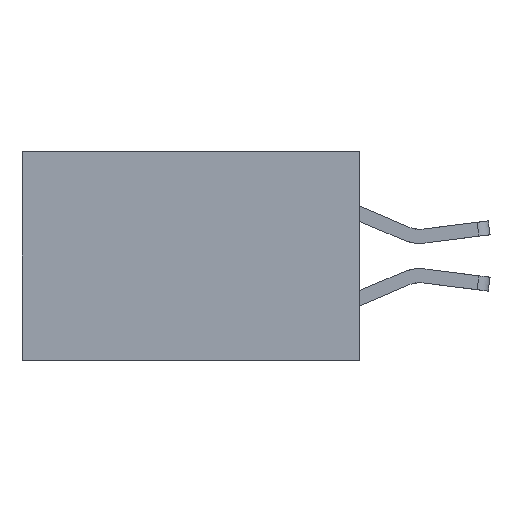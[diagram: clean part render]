
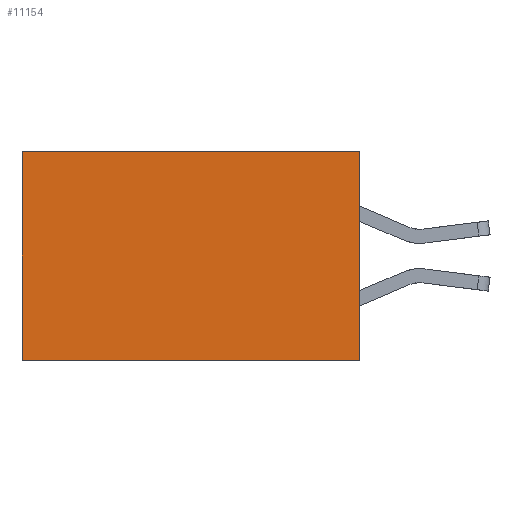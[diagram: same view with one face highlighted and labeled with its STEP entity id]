
A CAD part, left-side view. The second image highlights one B-rep face of the part: STEP entity #11154.
In plain terms, the highlighted planar face has unit normal (-1, 0, 0).
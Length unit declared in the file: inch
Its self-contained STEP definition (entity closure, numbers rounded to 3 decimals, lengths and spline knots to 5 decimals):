
#150 = DIRECTION ( 'NONE',  ( 0., 0., -1. ) ) ;
#681 = EDGE_LOOP ( 'NONE', ( #3591, #5218, #7576, #5569 ) ) ;
#901 = CARTESIAN_POINT ( 'NONE',  ( 0.2875, 0., 0. ) ) ;
#1009 = CARTESIAN_POINT ( 'NONE',  ( 0.2875, 0., 0. ) ) ;
#1150 = VECTOR ( 'NONE', #8488, 39.37008 ) ;
#2266 = DIRECTION ( 'NONE',  ( 0., 0., -1. ) ) ;
#2392 = VECTOR ( 'NONE', #3498, 39.37008 ) ;
#3498 = DIRECTION ( 'NONE',  ( 0., 1., 0. ) ) ;
#3591 = ORIENTED_EDGE ( 'NONE', *, *, #5013, .T. ) ;
#4480 = CARTESIAN_POINT ( 'NONE',  ( 0.2875, 0., -0.37 ) ) ;
#4952 = VERTEX_POINT ( 'NONE', #4480 ) ;
#5013 = EDGE_CURVE ( 'NONE', #6697, #14287, #14569, .T. ) ;
#5218 = ORIENTED_EDGE ( 'NONE', *, *, #15035, .F. ) ;
#5569 = ORIENTED_EDGE ( 'NONE', *, *, #9797, .T. ) ;
#5735 = LINE ( 'NONE', #8496, #11167 ) ;
#6097 = LINE ( 'NONE', #9530, #2392 ) ;
#6520 = CARTESIAN_POINT ( 'NONE',  ( 0.2875, 0., 0. ) ) ;
#6697 = VERTEX_POINT ( 'NONE', #12392 ) ;
#6992 = EDGE_CURVE ( 'NONE', #13157, #4952, #11507, .T. ) ;
#7576 = ORIENTED_EDGE ( 'NONE', *, *, #6992, .F. ) ;
#7700 = DIRECTION ( 'NONE',  ( 1., 0., 0. ) ) ;
#8488 = DIRECTION ( 'NONE',  ( 0., 0., -1. ) ) ;
#8496 = CARTESIAN_POINT ( 'NONE',  ( 0.2875, 0., -0.37 ) ) ;
#9530 = CARTESIAN_POINT ( 'NONE',  ( 0.2875, 0., 0. ) ) ;
#9797 = EDGE_CURVE ( 'NONE', #13157, #6697, #6097, .T. ) ;
#10917 = AXIS2_PLACEMENT_3D ( 'NONE', #6520, #7700, #150 ) ;
#11154 = ADVANCED_FACE ( 'NONE', ( #13433 ), #13381, .F. ) ;
#11167 = VECTOR ( 'NONE', #14165, 39.37008 ) ;
#11507 = LINE ( 'NONE', #901, #14167 ) ;
#11859 = CARTESIAN_POINT ( 'NONE',  ( 0.2875, 0.6, 0. ) ) ;
#12392 = CARTESIAN_POINT ( 'NONE',  ( 0.2875, 0.6, 0. ) ) ;
#13157 = VERTEX_POINT ( 'NONE', #1009 ) ;
#13381 = PLANE ( 'NONE',  #10917 ) ;
#13433 = FACE_OUTER_BOUND ( 'NONE', #681, .T. ) ;
#13881 = CARTESIAN_POINT ( 'NONE',  ( 0.2875, 0.6, -0.37 ) ) ;
#14165 = DIRECTION ( 'NONE',  ( 0., 1., 0. ) ) ;
#14167 = VECTOR ( 'NONE', #2266, 39.37008 ) ;
#14287 = VERTEX_POINT ( 'NONE', #13881 ) ;
#14569 = LINE ( 'NONE', #11859, #1150 ) ;
#15035 = EDGE_CURVE ( 'NONE', #4952, #14287, #5735, .T. ) ;
